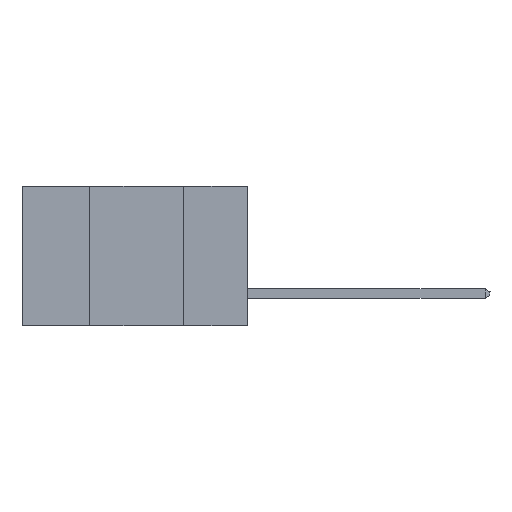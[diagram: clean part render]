
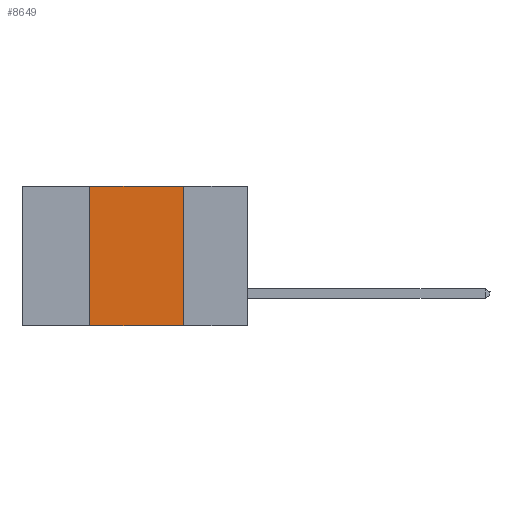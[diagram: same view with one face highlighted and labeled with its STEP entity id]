
A CAD part, left-side view. The second image highlights one B-rep face of the part: STEP entity #8649.
In plain terms, the highlighted planar face has unit normal (-1, 0, 0).
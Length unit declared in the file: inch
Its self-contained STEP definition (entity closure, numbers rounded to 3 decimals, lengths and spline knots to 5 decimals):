
#104 = EDGE_CURVE ( 'NONE', #9164, #2462, #5958, .T. ) ;
#524 = FACE_OUTER_BOUND ( 'NONE', #1686, .T. ) ;
#625 = CARTESIAN_POINT ( 'NONE',  ( 0., 0.42, -0.37 ) ) ;
#1626 = ORIENTED_EDGE ( 'NONE', *, *, #3597, .F. ) ;
#1686 = EDGE_LOOP ( 'NONE', ( #1626, #1740, #1826, #1865 ) ) ;
#1740 = ORIENTED_EDGE ( 'NONE', *, *, #2332, .F. ) ;
#1826 = ORIENTED_EDGE ( 'NONE', *, *, #104, .F. ) ;
#1865 = ORIENTED_EDGE ( 'NONE', *, *, #9559, .T. ) ;
#1875 = CARTESIAN_POINT ( 'NONE',  ( 0., 0.17, 0. ) ) ;
#2332 = EDGE_CURVE ( 'NONE', #2462, #3401, #6478, .T. ) ;
#2462 = VERTEX_POINT ( 'NONE', #8491 ) ;
#2526 = DIRECTION ( 'NONE',  ( 0., 0., 1. ) ) ;
#2862 = LINE ( 'NONE', #8968, #8582 ) ;
#3355 = DIRECTION ( 'NONE',  ( 1., 0., 0. ) ) ;
#3401 = VERTEX_POINT ( 'NONE', #1875 ) ;
#3597 = EDGE_CURVE ( 'NONE', #3401, #7425, #8906, .T. ) ;
#3797 = DIRECTION ( 'NONE',  ( 0., -1., 0. ) ) ;
#5958 = LINE ( 'NONE', #8508, #7361 ) ;
#5959 = CARTESIAN_POINT ( 'NONE',  ( 0., 0.17, -0.37 ) ) ;
#6478 = LINE ( 'NONE', #8683, #8157 ) ;
#7006 = VECTOR ( 'NONE', #7614, 39.37008 ) ;
#7116 = PLANE ( 'NONE',  #9296 ) ;
#7361 = VECTOR ( 'NONE', #2526, 39.37008 ) ;
#7425 = VERTEX_POINT ( 'NONE', #5959 ) ;
#7614 = DIRECTION ( 'NONE',  ( 0., 0., -1. ) ) ;
#7827 = CARTESIAN_POINT ( 'NONE',  ( 0., 0.6, 0. ) ) ;
#8157 = VECTOR ( 'NONE', #8646, 39.37008 ) ;
#8236 = CARTESIAN_POINT ( 'NONE',  ( 0., 0.17, 0. ) ) ;
#8491 = CARTESIAN_POINT ( 'NONE',  ( 0., 0.42, 0. ) ) ;
#8508 = CARTESIAN_POINT ( 'NONE',  ( 0., 0.42, 0. ) ) ;
#8567 = DIRECTION ( 'NONE',  ( 0., 0., -1. ) ) ;
#8582 = VECTOR ( 'NONE', #3797, 39.37008 ) ;
#8646 = DIRECTION ( 'NONE',  ( 0., -1., 0. ) ) ;
#8649 = ADVANCED_FACE ( 'NONE', ( #524 ), #7116, .F. ) ;
#8683 = CARTESIAN_POINT ( 'NONE',  ( 0., 0.6, 0. ) ) ;
#8906 = LINE ( 'NONE', #8236, #7006 ) ;
#8968 = CARTESIAN_POINT ( 'NONE',  ( 0., 0.6, -0.37 ) ) ;
#9164 = VERTEX_POINT ( 'NONE', #625 ) ;
#9296 = AXIS2_PLACEMENT_3D ( 'NONE', #7827, #3355, #8567 ) ;
#9559 = EDGE_CURVE ( 'NONE', #9164, #7425, #2862, .T. ) ;
